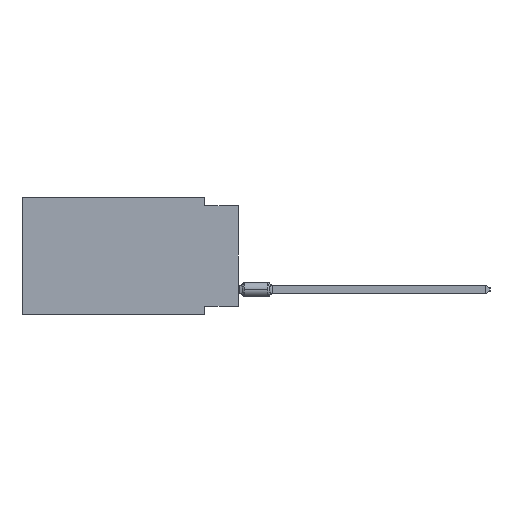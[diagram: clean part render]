
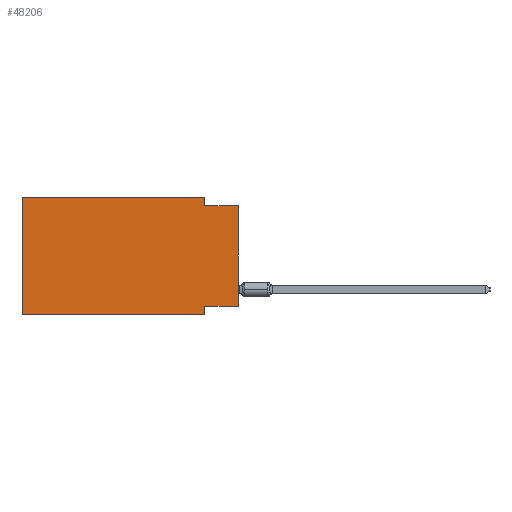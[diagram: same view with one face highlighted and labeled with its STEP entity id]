
A CAD part, left-side view. The second image highlights one B-rep face of the part: STEP entity #48206.
In plain terms, the highlighted planar face has unit normal (-1, 0, 0).
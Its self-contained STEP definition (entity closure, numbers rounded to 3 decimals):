
#569 = AXIS2_PLACEMENT_3D ( 'NONE', #80193, #40618, #16189 ) ;
#4844 = LINE ( 'NONE', #81139, #61153 ) ;
#5322 = CARTESIAN_POINT ( 'NONE',  ( 0., 16.383, -8.89 ) ) ;
#6394 = LINE ( 'NONE', #5322, #82592 ) ;
#7276 = EDGE_CURVE ( 'NONE', #62460, #19967, #6394, .T. ) ;
#7494 = LINE ( 'NONE', #106690, #44440 ) ;
#13262 = DIRECTION ( 'NONE',  ( 0., 0., 1. ) ) ;
#15142 = CARTESIAN_POINT ( 'NONE',  ( 0., 16.383, 0. ) ) ;
#16177 = DIRECTION ( 'NONE',  ( 0., 1., 0. ) ) ;
#16189 = DIRECTION ( 'NONE',  ( 0., 0., -1. ) ) ;
#19699 = ORIENTED_EDGE ( 'NONE', *, *, #7276, .T. ) ;
#19967 = VERTEX_POINT ( 'NONE', #49864 ) ;
#20964 = VERTEX_POINT ( 'NONE', #86248 ) ;
#22281 = ORIENTED_EDGE ( 'NONE', *, *, #63512, .F. ) ;
#22541 = EDGE_CURVE ( 'NONE', #60137, #20964, #75498, .T. ) ;
#22716 = FACE_OUTER_BOUND ( 'NONE', #77075, .T. ) ;
#27968 = ORIENTED_EDGE ( 'NONE', *, *, #52383, .F. ) ;
#32481 = DIRECTION ( 'NONE',  ( 0., 0., -1. ) ) ;
#36326 = CARTESIAN_POINT ( 'NONE',  ( 0., 0., 0. ) ) ;
#36617 = CARTESIAN_POINT ( 'NONE',  ( 0., 2.54, -8.89 ) ) ;
#38158 = ORIENTED_EDGE ( 'NONE', *, *, #52122, .F. ) ;
#39638 = VERTEX_POINT ( 'NONE', #98017 ) ;
#40558 = EDGE_CURVE ( 'NONE', #62460, #80821, #97754, .T. ) ;
#40618 = DIRECTION ( 'NONE',  ( 1., 0., 0. ) ) ;
#42232 = VECTOR ( 'NONE', #69649, 1000. ) ;
#44091 = CARTESIAN_POINT ( 'NONE',  ( 0., 16.383, 0. ) ) ;
#44440 = VECTOR ( 'NONE', #32481, 1000. ) ;
#48206 = ADVANCED_FACE ( 'NONE', ( #22716 ), #89939, .F. ) ;
#49864 = CARTESIAN_POINT ( 'NONE',  ( 0., 2.54, -8.89 ) ) ;
#50235 = VECTOR ( 'NONE', #86145, 1000. ) ;
#50468 = CARTESIAN_POINT ( 'NONE',  ( 0., 2.54, -0.635 ) ) ;
#51170 = DIRECTION ( 'NONE',  ( 0., -1., 0. ) ) ;
#51714 = LINE ( 'NONE', #44091, #107142 ) ;
#52122 = EDGE_CURVE ( 'NONE', #74886, #20964, #4844, .T. ) ;
#52383 = EDGE_CURVE ( 'NONE', #39638, #19967, #77805, .T. ) ;
#56733 = DIRECTION ( 'NONE',  ( 0., -1., 0. ) ) ;
#57079 = ORIENTED_EDGE ( 'NONE', *, *, #40558, .F. ) ;
#57399 = CARTESIAN_POINT ( 'NONE',  ( 0., 0., -8.255 ) ) ;
#60137 = VERTEX_POINT ( 'NONE', #71743 ) ;
#61153 = VECTOR ( 'NONE', #56733, 1000. ) ;
#62460 = VERTEX_POINT ( 'NONE', #69783 ) ;
#63512 = EDGE_CURVE ( 'NONE', #60137, #39638, #67670, .T. ) ;
#67670 = LINE ( 'NONE', #57399, #81610 ) ;
#69366 = ORIENTED_EDGE ( 'NONE', *, *, #22541, .T. ) ;
#69649 = DIRECTION ( 'NONE',  ( 0., 0., -1. ) ) ;
#69783 = CARTESIAN_POINT ( 'NONE',  ( 0., 16.383, -8.89 ) ) ;
#71743 = CARTESIAN_POINT ( 'NONE',  ( 0., 0., -8.255 ) ) ;
#72557 = DIRECTION ( 'NONE',  ( 0., -1., 0. ) ) ;
#74886 = VERTEX_POINT ( 'NONE', #50468 ) ;
#75498 = LINE ( 'NONE', #36326, #50235 ) ;
#77075 = EDGE_LOOP ( 'NONE', ( #69366, #38158, #78248, #93057, #57079, #19699, #27968, #22281 ) ) ;
#77805 = LINE ( 'NONE', #36617, #42232 ) ;
#78238 = EDGE_CURVE ( 'NONE', #103027, #74886, #7494, .T. ) ;
#78248 = ORIENTED_EDGE ( 'NONE', *, *, #78238, .F. ) ;
#80193 = CARTESIAN_POINT ( 'NONE',  ( 0., 16.383, 0. ) ) ;
#80465 = CARTESIAN_POINT ( 'NONE',  ( 0., 16.383, 0. ) ) ;
#80821 = VERTEX_POINT ( 'NONE', #15142 ) ;
#81139 = CARTESIAN_POINT ( 'NONE',  ( 0., 0., -0.635 ) ) ;
#81610 = VECTOR ( 'NONE', #16177, 1000. ) ;
#82592 = VECTOR ( 'NONE', #72557, 1000. ) ;
#85991 = VECTOR ( 'NONE', #13262, 1000. ) ;
#86145 = DIRECTION ( 'NONE',  ( 0., 0., 1. ) ) ;
#86248 = CARTESIAN_POINT ( 'NONE',  ( 0., 0., -0.635 ) ) ;
#89939 = PLANE ( 'NONE',  #569 ) ;
#93057 = ORIENTED_EDGE ( 'NONE', *, *, #95767, .F. ) ;
#95767 = EDGE_CURVE ( 'NONE', #80821, #103027, #51714, .T. ) ;
#97754 = LINE ( 'NONE', #80465, #85991 ) ;
#97889 = CARTESIAN_POINT ( 'NONE',  ( 0., 2.54, 0. ) ) ;
#98017 = CARTESIAN_POINT ( 'NONE',  ( 0., 2.54, -8.255 ) ) ;
#103027 = VERTEX_POINT ( 'NONE', #97889 ) ;
#106690 = CARTESIAN_POINT ( 'NONE',  ( 0., 2.54, 0. ) ) ;
#107142 = VECTOR ( 'NONE', #51170, 1000. ) ;
